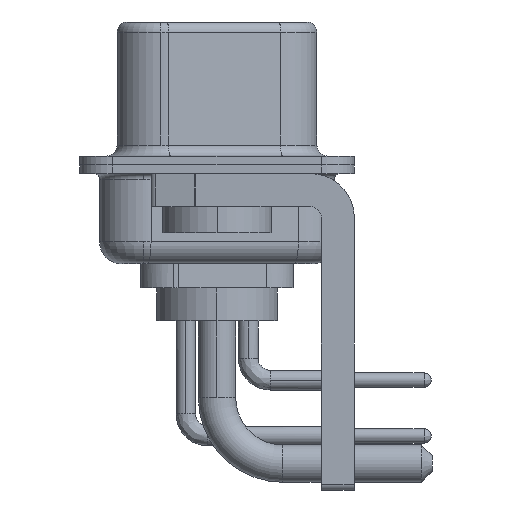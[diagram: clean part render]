
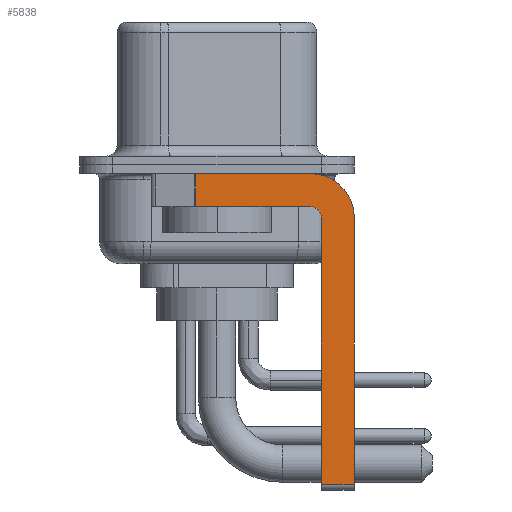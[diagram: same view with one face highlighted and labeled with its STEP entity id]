
A CAD part, left-side view. The second image highlights one B-rep face of the part: STEP entity #5838.
In plain terms, the highlighted planar face has unit normal (-1, 0, 0).
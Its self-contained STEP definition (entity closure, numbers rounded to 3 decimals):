
#491 = LINE ( 'NONE', #6935, #9939 ) ;
#622 = LINE ( 'NONE', #2518, #1266 ) ;
#1266 = VECTOR ( 'NONE', #9249, 1000. ) ;
#1329 = ORIENTED_EDGE ( 'NONE', *, *, #24861, .F. ) ;
#1383 = VECTOR ( 'NONE', #22675, 1000. ) ;
#2518 = CARTESIAN_POINT ( 'NONE',  ( -2.9, 0.978, -1.9 ) ) ;
#2633 = CARTESIAN_POINT ( 'NONE',  ( -2.9, 3., -0.4 ) ) ;
#3095 = DIRECTION ( 'NONE',  ( 0., -1., 0. ) ) ;
#3705 = FACE_OUTER_BOUND ( 'NONE', #11772, .T. ) ;
#4605 = CIRCLE ( 'NONE', #12990, 0.5 ) ;
#4710 = EDGE_CURVE ( 'NONE', #14049, #8610, #4605, .T. ) ;
#4937 = CARTESIAN_POINT ( 'NONE',  ( -2.9, -4.25, -1.9 ) ) ;
#5332 = VERTEX_POINT ( 'NONE', #25834 ) ;
#5838 = ADVANCED_FACE ( 'NONE', ( #3705 ), #12616, .F. ) ;
#6031 = CARTESIAN_POINT ( 'NONE',  ( -2.9, -4.25, -1.9 ) ) ;
#6102 = CARTESIAN_POINT ( 'NONE',  ( -2.9, -4.75, -14.55 ) ) ;
#6179 = ORIENTED_EDGE ( 'NONE', *, *, #9961, .F. ) ;
#6869 = LINE ( 'NONE', #24688, #20941 ) ;
#6935 = CARTESIAN_POINT ( 'NONE',  ( -2.9, -4.75, -14.8 ) ) ;
#6989 = DIRECTION ( 'NONE',  ( 0., 0., 1. ) ) ;
#7233 = DIRECTION ( 'NONE',  ( 0., 0., 1. ) ) ;
#7356 = LINE ( 'NONE', #20501, #19462 ) ;
#7760 = CARTESIAN_POINT ( 'NONE',  ( -2.9, -6.25, -2.4 ) ) ;
#8610 = VERTEX_POINT ( 'NONE', #4937 ) ;
#8647 = CARTESIAN_POINT ( 'NONE',  ( -2.9, 0.978, -1.9 ) ) ;
#9170 = DIRECTION ( 'NONE',  ( -1., 0., 0. ) ) ;
#9249 = DIRECTION ( 'NONE',  ( 0., 0., -1. ) ) ;
#9289 = CARTESIAN_POINT ( 'NONE',  ( -2.9, -4.75, -2.4 ) ) ;
#9462 = ORIENTED_EDGE ( 'NONE', *, *, #9675, .F. ) ;
#9509 = EDGE_CURVE ( 'NONE', #11299, #5332, #6869, .T. ) ;
#9675 = EDGE_CURVE ( 'NONE', #8610, #25382, #19028, .T. ) ;
#9883 = CARTESIAN_POINT ( 'NONE',  ( -2.9, -4.25, -0.4 ) ) ;
#9939 = VECTOR ( 'NONE', #7233, 1000. ) ;
#9961 = EDGE_CURVE ( 'NONE', #23961, #25659, #13763, .T. ) ;
#11299 = VERTEX_POINT ( 'NONE', #7760 ) ;
#11772 = EDGE_LOOP ( 'NONE', ( #6179, #24013, #9462, #23466, #22927, #20239, #17349, #1329 ) ) ;
#12616 = PLANE ( 'NONE',  #27036 ) ;
#12990 = AXIS2_PLACEMENT_3D ( 'NONE', #24520, #9170, #6989 ) ;
#13763 = LINE ( 'NONE', #2633, #1383 ) ;
#14013 = VERTEX_POINT ( 'NONE', #6102 ) ;
#14049 = VERTEX_POINT ( 'NONE', #9289 ) ;
#15056 = CARTESIAN_POINT ( 'NONE',  ( -2.9, -4.25, -2.4 ) ) ;
#16815 = DIRECTION ( 'NONE',  ( 1., 0., 0. ) ) ;
#17143 = DIRECTION ( 'NONE',  ( 0., 0., -1. ) ) ;
#17349 = ORIENTED_EDGE ( 'NONE', *, *, #9509, .F. ) ;
#18825 = AXIS2_PLACEMENT_3D ( 'NONE', #15056, #16815, #23544 ) ;
#19028 = LINE ( 'NONE', #6031, #26080 ) ;
#19317 = EDGE_CURVE ( 'NONE', #14013, #5332, #7356, .T. ) ;
#19320 = EDGE_CURVE ( 'NONE', #23961, #25382, #622, .T. ) ;
#19462 = VECTOR ( 'NONE', #3095, 1000. ) ;
#20239 = ORIENTED_EDGE ( 'NONE', *, *, #19317, .T. ) ;
#20501 = CARTESIAN_POINT ( 'NONE',  ( -2.9, -4.25, -14.55 ) ) ;
#20941 = VECTOR ( 'NONE', #27157, 1000. ) ;
#21531 = CARTESIAN_POINT ( 'NONE',  ( -2.9, -4.25, -2.4 ) ) ;
#22675 = DIRECTION ( 'NONE',  ( 0., -1., 0. ) ) ;
#22927 = ORIENTED_EDGE ( 'NONE', *, *, #24123, .F. ) ;
#23173 = CARTESIAN_POINT ( 'NONE',  ( -2.9, 0.978, -0.4 ) ) ;
#23466 = ORIENTED_EDGE ( 'NONE', *, *, #4710, .F. ) ;
#23544 = DIRECTION ( 'NONE',  ( 0., 0., -1. ) ) ;
#23961 = VERTEX_POINT ( 'NONE', #23173 ) ;
#24013 = ORIENTED_EDGE ( 'NONE', *, *, #19320, .T. ) ;
#24123 = EDGE_CURVE ( 'NONE', #14013, #14049, #491, .T. ) ;
#24520 = CARTESIAN_POINT ( 'NONE',  ( -2.9, -4.25, -2.4 ) ) ;
#24688 = CARTESIAN_POINT ( 'NONE',  ( -2.9, -6.25, -2.4 ) ) ;
#24861 = EDGE_CURVE ( 'NONE', #25659, #11299, #27671, .T. ) ;
#25382 = VERTEX_POINT ( 'NONE', #8647 ) ;
#25659 = VERTEX_POINT ( 'NONE', #9883 ) ;
#25834 = CARTESIAN_POINT ( 'NONE',  ( -2.9, -6.25, -14.55 ) ) ;
#26080 = VECTOR ( 'NONE', #26176, 1000. ) ;
#26176 = DIRECTION ( 'NONE',  ( 0., 1., 0. ) ) ;
#27036 = AXIS2_PLACEMENT_3D ( 'NONE', #21531, #28359, #17143 ) ;
#27157 = DIRECTION ( 'NONE',  ( 0., 0., -1. ) ) ;
#27671 = CIRCLE ( 'NONE', #18825, 2. ) ;
#28359 = DIRECTION ( 'NONE',  ( 1., 0., 0. ) ) ;
